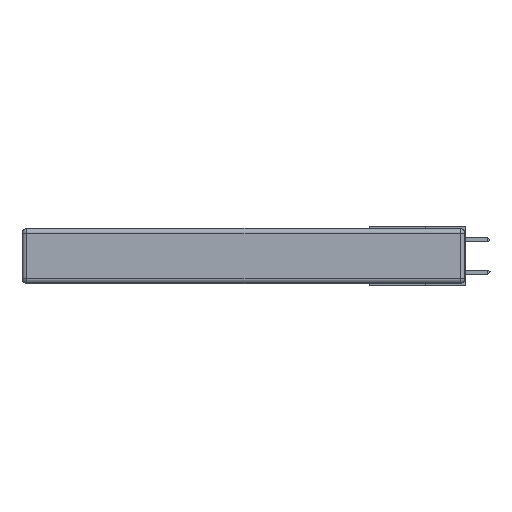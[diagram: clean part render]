
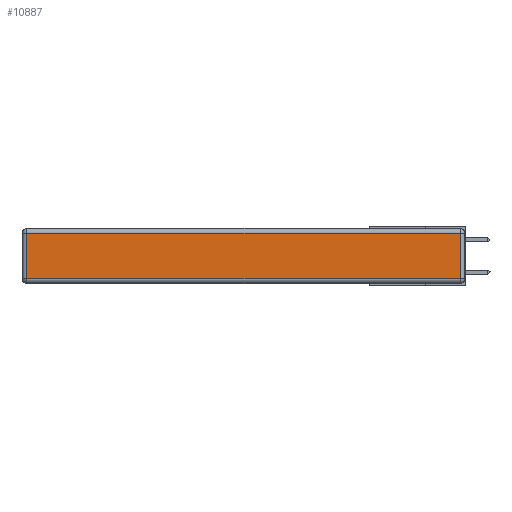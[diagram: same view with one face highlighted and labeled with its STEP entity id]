
A CAD part, left-side view. The second image highlights one B-rep face of the part: STEP entity #10887.
In plain terms, the highlighted planar face has unit normal (-1, 0, 0).
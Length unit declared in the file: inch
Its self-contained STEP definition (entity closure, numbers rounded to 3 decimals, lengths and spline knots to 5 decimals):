
#65 = DIRECTION ( 'NONE',  ( 0., -1., 0. ) ) ;
#123 = CARTESIAN_POINT ( 'NONE',  ( 0., 0.03, -0.03 ) ) ;
#538 = DIRECTION ( 'NONE',  ( 0., 0., 1. ) ) ;
#3426 = VECTOR ( 'NONE', #65, 39.37008 ) ;
#4133 = ORIENTED_EDGE ( 'NONE', *, *, #12304, .T. ) ;
#4696 = LINE ( 'NONE', #7749, #12558 ) ;
#4729 = CARTESIAN_POINT ( 'NONE',  ( 0., 0.03, -0.313 ) ) ;
#5427 = LINE ( 'NONE', #18504, #13721 ) ;
#5790 = FACE_OUTER_BOUND ( 'NONE', #17587, .T. ) ;
#6251 = CARTESIAN_POINT ( 'NONE',  ( 0., 0., -0.343 ) ) ;
#6376 = EDGE_CURVE ( 'NONE', #14661, #18191, #8908, .T. ) ;
#6862 = DIRECTION ( 'NONE',  ( 0., 1., 0. ) ) ;
#7690 = DIRECTION ( 'NONE',  ( 0., 0., -1. ) ) ;
#7749 = CARTESIAN_POINT ( 'NONE',  ( 0., 2.72, -0.343 ) ) ;
#8188 = CARTESIAN_POINT ( 'NONE',  ( 0., 0.03, -0.343 ) ) ;
#8579 = LINE ( 'NONE', #15799, #3426 ) ;
#8908 = LINE ( 'NONE', #8188, #18297 ) ;
#9440 = DIRECTION ( 'NONE',  ( -1., 0., 0. ) ) ;
#10887 = ADVANCED_FACE ( 'NONE', ( #5790 ), #10952, .T. ) ;
#10952 = PLANE ( 'NONE',  #17200 ) ;
#11292 = VERTEX_POINT ( 'NONE', #13159 ) ;
#12304 = EDGE_CURVE ( 'NONE', #17222, #14661, #8579, .T. ) ;
#12558 = VECTOR ( 'NONE', #7690, 39.37008 ) ;
#12675 = EDGE_CURVE ( 'NONE', #18191, #11292, #5427, .T. ) ;
#13159 = CARTESIAN_POINT ( 'NONE',  ( 0., 2.72, -0.03 ) ) ;
#13721 = VECTOR ( 'NONE', #6862, 39.37008 ) ;
#14038 = ORIENTED_EDGE ( 'NONE', *, *, #12675, .T. ) ;
#14485 = CARTESIAN_POINT ( 'NONE',  ( 0., 2.72, -0.313 ) ) ;
#14578 = EDGE_CURVE ( 'NONE', #11292, #17222, #4696, .T. ) ;
#14661 = VERTEX_POINT ( 'NONE', #4729 ) ;
#15799 = CARTESIAN_POINT ( 'NONE',  ( 0., 0., -0.313 ) ) ;
#16284 = ORIENTED_EDGE ( 'NONE', *, *, #6376, .T. ) ;
#16685 = DIRECTION ( 'NONE',  ( 0., 0., 1. ) ) ;
#17200 = AXIS2_PLACEMENT_3D ( 'NONE', #6251, #9440, #538 ) ;
#17222 = VERTEX_POINT ( 'NONE', #14485 ) ;
#17587 = EDGE_LOOP ( 'NONE', ( #4133, #16284, #14038, #18012 ) ) ;
#18012 = ORIENTED_EDGE ( 'NONE', *, *, #14578, .T. ) ;
#18191 = VERTEX_POINT ( 'NONE', #123 ) ;
#18297 = VECTOR ( 'NONE', #16685, 39.37008 ) ;
#18504 = CARTESIAN_POINT ( 'NONE',  ( 0., 2.75, -0.03 ) ) ;
